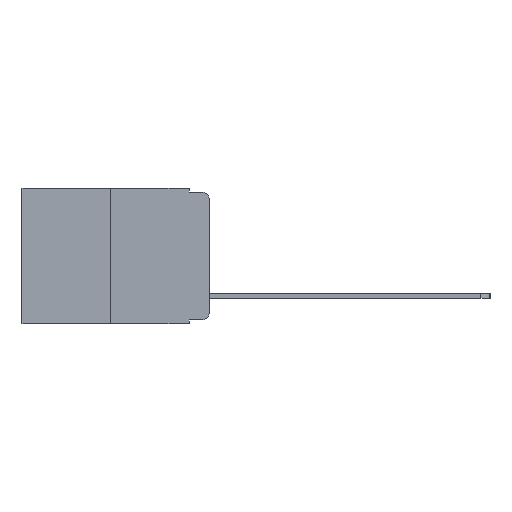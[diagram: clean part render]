
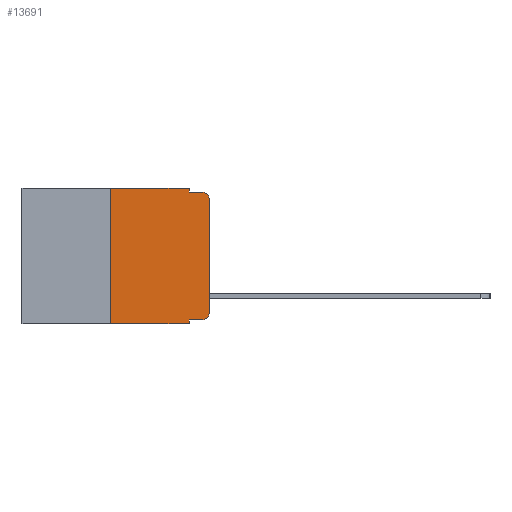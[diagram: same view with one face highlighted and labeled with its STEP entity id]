
A CAD part, left-side view. The second image highlights one B-rep face of the part: STEP entity #13691.
In plain terms, the highlighted planar face has unit normal (-1, 0, 0).
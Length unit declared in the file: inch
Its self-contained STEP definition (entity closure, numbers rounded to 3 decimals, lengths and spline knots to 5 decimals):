
#540 = EDGE_CURVE ( 'NONE', #3730, #13342, #6150, .T. ) ;
#819 = ORIENTED_EDGE ( 'NONE', *, *, #17025, .T. ) ;
#1103 = LINE ( 'NONE', #7259, #17002 ) ;
#1121 = CIRCLE ( 'NONE', #15162, 0.02 ) ;
#1309 = CARTESIAN_POINT ( 'NONE',  ( 0., 0.051, -0.01 ) ) ;
#1368 = ORIENTED_EDGE ( 'NONE', *, *, #16084, .F. ) ;
#1448 = DIRECTION ( 'NONE',  ( 0., -1., 0. ) ) ;
#1954 = VECTOR ( 'NONE', #12039, 39.37008 ) ;
#2111 = VERTEX_POINT ( 'NONE', #12834 ) ;
#2427 = ORIENTED_EDGE ( 'NONE', *, *, #10641, .F. ) ;
#2901 = CARTESIAN_POINT ( 'NONE',  ( 0., 0.25, 0. ) ) ;
#3319 = VERTEX_POINT ( 'NONE', #11606 ) ;
#3429 = LINE ( 'NONE', #4871, #14777 ) ;
#3463 = ORIENTED_EDGE ( 'NONE', *, *, #12199, .F. ) ;
#3730 = VERTEX_POINT ( 'NONE', #17007 ) ;
#4057 = VECTOR ( 'NONE', #17186, 39.37008 ) ;
#4430 = LINE ( 'NONE', #1309, #8371 ) ;
#4460 = ORIENTED_EDGE ( 'NONE', *, *, #7349, .T. ) ;
#4814 = CARTESIAN_POINT ( 'NONE',  ( 0., 0.051, -0.01 ) ) ;
#4871 = CARTESIAN_POINT ( 'NONE',  ( 0., 0.051, -0.333 ) ) ;
#4913 = CIRCLE ( 'NONE', #9876, 0.02 ) ;
#5307 = VERTEX_POINT ( 'NONE', #9520 ) ;
#5366 = VERTEX_POINT ( 'NONE', #12360 ) ;
#5870 = VECTOR ( 'NONE', #1448, 39.37008 ) ;
#6128 = DIRECTION ( 'NONE',  ( -1., 0., 0. ) ) ;
#6150 = LINE ( 'NONE', #16355, #1954 ) ;
#6320 = FACE_OUTER_BOUND ( 'NONE', #14202, .T. ) ;
#7106 = CARTESIAN_POINT ( 'NONE',  ( 0., 0.473, 0. ) ) ;
#7259 = CARTESIAN_POINT ( 'NONE',  ( 0., 0.25, 0. ) ) ;
#7308 = CARTESIAN_POINT ( 'NONE',  ( 0., 0.473, 0. ) ) ;
#7349 = EDGE_CURVE ( 'NONE', #5307, #3730, #1121, .T. ) ;
#7519 = ORIENTED_EDGE ( 'NONE', *, *, #8200, .T. ) ;
#7902 = DIRECTION ( 'NONE',  ( -1., 0., 0. ) ) ;
#8146 = CARTESIAN_POINT ( 'NONE',  ( 0., 0.02, -0.01 ) ) ;
#8200 = EDGE_CURVE ( 'NONE', #3319, #5366, #8827, .T. ) ;
#8300 = EDGE_CURVE ( 'NONE', #2111, #5307, #3429, .T. ) ;
#8371 = VECTOR ( 'NONE', #14887, 39.37008 ) ;
#8538 = DIRECTION ( 'NONE',  ( 0., 0., -1. ) ) ;
#8618 = ORIENTED_EDGE ( 'NONE', *, *, #540, .T. ) ;
#8827 = LINE ( 'NONE', #17771, #5870 ) ;
#9056 = CARTESIAN_POINT ( 'NONE',  ( 0., 0.051, 0. ) ) ;
#9520 = CARTESIAN_POINT ( 'NONE',  ( 0., 0.02, -0.333 ) ) ;
#9876 = AXIS2_PLACEMENT_3D ( 'NONE', #16579, #7902, #18010 ) ;
#9937 = CARTESIAN_POINT ( 'NONE',  ( 0., 0.051, 0. ) ) ;
#10010 = ORIENTED_EDGE ( 'NONE', *, *, #13199, .F. ) ;
#10211 = LINE ( 'NONE', #9056, #17444 ) ;
#10530 = DIRECTION ( 'NONE',  ( 0., 0., -1. ) ) ;
#10641 = EDGE_CURVE ( 'NONE', #13823, #18740, #18000, .T. ) ;
#10768 = DIRECTION ( 'NONE',  ( 0., -1., 0. ) ) ;
#11233 = EDGE_CURVE ( 'NONE', #2111, #5366, #11878, .T. ) ;
#11409 = PLANE ( 'NONE',  #17941 ) ;
#11606 = CARTESIAN_POINT ( 'NONE',  ( 0., 0.25, -0.343 ) ) ;
#11878 = LINE ( 'NONE', #9937, #4057 ) ;
#12039 = DIRECTION ( 'NONE',  ( 0., 0., 1. ) ) ;
#12199 = EDGE_CURVE ( 'NONE', #3319, #13823, #1103, .T. ) ;
#12310 = CARTESIAN_POINT ( 'NONE',  ( 0., 0., -0.03 ) ) ;
#12360 = CARTESIAN_POINT ( 'NONE',  ( 0., 0.051, -0.343 ) ) ;
#12834 = CARTESIAN_POINT ( 'NONE',  ( 0., 0.051, -0.333 ) ) ;
#13144 = DIRECTION ( 'NONE',  ( 0., -1., 0. ) ) ;
#13199 = EDGE_CURVE ( 'NONE', #18740, #18915, #10211, .T. ) ;
#13342 = VERTEX_POINT ( 'NONE', #12310 ) ;
#13691 = ADVANCED_FACE ( 'NONE', ( #6320 ), #11409, .F. ) ;
#13823 = VERTEX_POINT ( 'NONE', #2901 ) ;
#14202 = EDGE_LOOP ( 'NONE', ( #8618, #819, #1368, #10010, #2427, #3463, #7519, #15251, #18970, #4460 ) ) ;
#14777 = VECTOR ( 'NONE', #10768, 39.37008 ) ;
#14887 = DIRECTION ( 'NONE',  ( 0., -1., 0. ) ) ;
#14888 = CARTESIAN_POINT ( 'NONE',  ( 0., 0.02, -0.313 ) ) ;
#15162 = AXIS2_PLACEMENT_3D ( 'NONE', #14888, #6128, #16294 ) ;
#15251 = ORIENTED_EDGE ( 'NONE', *, *, #11233, .F. ) ;
#15613 = CARTESIAN_POINT ( 'NONE',  ( 0., 0.051, 0. ) ) ;
#16084 = EDGE_CURVE ( 'NONE', #18915, #17837, #4430, .T. ) ;
#16294 = DIRECTION ( 'NONE',  ( 0., 0., -1. ) ) ;
#16355 = CARTESIAN_POINT ( 'NONE',  ( 0., 0., 0. ) ) ;
#16579 = CARTESIAN_POINT ( 'NONE',  ( 0., 0.02, -0.03 ) ) ;
#17002 = VECTOR ( 'NONE', #17353, 39.37008 ) ;
#17007 = CARTESIAN_POINT ( 'NONE',  ( 0., 0., -0.313 ) ) ;
#17025 = EDGE_CURVE ( 'NONE', #13342, #17837, #4913, .T. ) ;
#17097 = VECTOR ( 'NONE', #13144, 39.37008 ) ;
#17186 = DIRECTION ( 'NONE',  ( 0., 0., -1. ) ) ;
#17203 = DIRECTION ( 'NONE',  ( 1., 0., 0. ) ) ;
#17353 = DIRECTION ( 'NONE',  ( 0., 0., 1. ) ) ;
#17444 = VECTOR ( 'NONE', #10530, 39.37008 ) ;
#17771 = CARTESIAN_POINT ( 'NONE',  ( 0., 0.473, -0.343 ) ) ;
#17837 = VERTEX_POINT ( 'NONE', #8146 ) ;
#17941 = AXIS2_PLACEMENT_3D ( 'NONE', #7106, #17203, #8538 ) ;
#18000 = LINE ( 'NONE', #7308, #17097 ) ;
#18010 = DIRECTION ( 'NONE',  ( 0., 0., -1. ) ) ;
#18740 = VERTEX_POINT ( 'NONE', #15613 ) ;
#18915 = VERTEX_POINT ( 'NONE', #4814 ) ;
#18970 = ORIENTED_EDGE ( 'NONE', *, *, #8300, .T. ) ;
